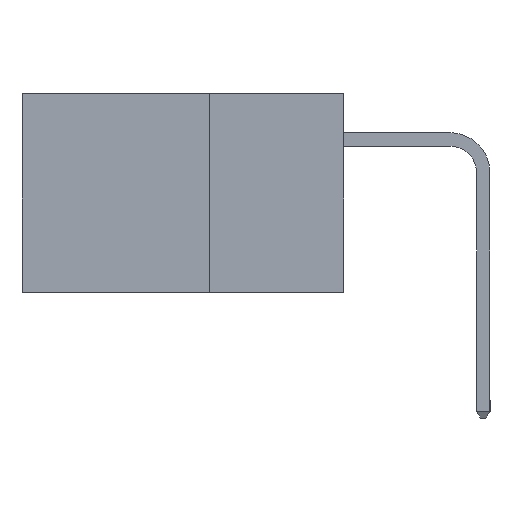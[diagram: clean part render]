
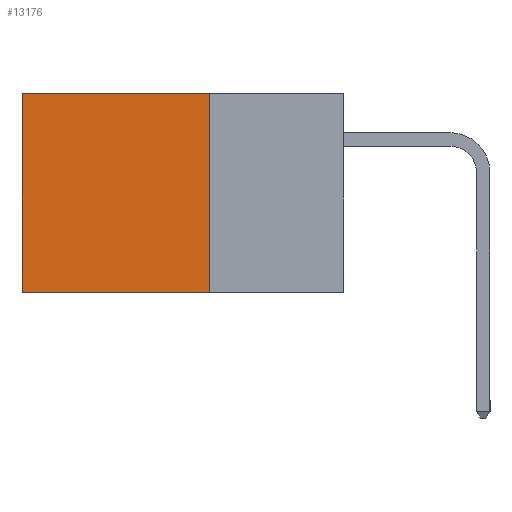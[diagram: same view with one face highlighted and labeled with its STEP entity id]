
A CAD part, left-side view. The second image highlights one B-rep face of the part: STEP entity #13176.
In plain terms, the highlighted planar face has unit normal (-1, 0, 0).
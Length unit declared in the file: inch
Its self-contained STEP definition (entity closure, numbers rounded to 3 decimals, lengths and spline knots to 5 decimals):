
#333 = CARTESIAN_POINT ( 'NONE',  ( 0.2615, 0.6, -0.37 ) ) ;
#347 = CARTESIAN_POINT ( 'NONE',  ( 0.2615, 0.25, 0. ) ) ;
#419 = DIRECTION ( 'NONE',  ( 0., 1., 0. ) ) ;
#1109 = DIRECTION ( 'NONE',  ( 1., 0., 0. ) ) ;
#2502 = VERTEX_POINT ( 'NONE', #6564 ) ;
#2642 = ORIENTED_EDGE ( 'NONE', *, *, #3732, .T. ) ;
#2700 = LINE ( 'NONE', #7761, #5968 ) ;
#2918 = VECTOR ( 'NONE', #11281, 39.37008 ) ;
#3124 = EDGE_CURVE ( 'NONE', #2502, #11687, #10125, .T. ) ;
#3251 = DIRECTION ( 'NONE',  ( 0., 0., -1. ) ) ;
#3732 = EDGE_CURVE ( 'NONE', #7903, #11687, #11468, .T. ) ;
#4304 = VECTOR ( 'NONE', #12937, 39.37008 ) ;
#5243 = PLANE ( 'NONE',  #12596 ) ;
#5786 = VECTOR ( 'NONE', #419, 39.37008 ) ;
#5968 = VECTOR ( 'NONE', #7655, 39.37008 ) ;
#6080 = CARTESIAN_POINT ( 'NONE',  ( 0.2615, 0.6, 0. ) ) ;
#6446 = CARTESIAN_POINT ( 'NONE',  ( 0.2615, 0.25, -0.37 ) ) ;
#6500 = ORIENTED_EDGE ( 'NONE', *, *, #3124, .F. ) ;
#6564 = CARTESIAN_POINT ( 'NONE',  ( 0.2615, 0.25, -0.37 ) ) ;
#7358 = EDGE_CURVE ( 'NONE', #10373, #2502, #2700, .T. ) ;
#7655 = DIRECTION ( 'NONE',  ( 0., 0., -1. ) ) ;
#7704 = FACE_OUTER_BOUND ( 'NONE', #12308, .T. ) ;
#7761 = CARTESIAN_POINT ( 'NONE',  ( 0.2615, 0.25, -0.37 ) ) ;
#7903 = VERTEX_POINT ( 'NONE', #6080 ) ;
#8422 = EDGE_CURVE ( 'NONE', #10373, #7903, #13322, .T. ) ;
#10125 = LINE ( 'NONE', #6446, #4304 ) ;
#10373 = VERTEX_POINT ( 'NONE', #11494 ) ;
#11281 = DIRECTION ( 'NONE',  ( 0., 0., -1. ) ) ;
#11468 = LINE ( 'NONE', #333, #2918 ) ;
#11494 = CARTESIAN_POINT ( 'NONE',  ( 0.2615, 0.25, 0. ) ) ;
#11687 = VERTEX_POINT ( 'NONE', #13494 ) ;
#12063 = ORIENTED_EDGE ( 'NONE', *, *, #8422, .T. ) ;
#12308 = EDGE_LOOP ( 'NONE', ( #2642, #6500, #12825, #12063 ) ) ;
#12596 = AXIS2_PLACEMENT_3D ( 'NONE', #12908, #1109, #3251 ) ;
#12825 = ORIENTED_EDGE ( 'NONE', *, *, #7358, .F. ) ;
#12908 = CARTESIAN_POINT ( 'NONE',  ( 0.2615, 0.25, -0.37 ) ) ;
#12937 = DIRECTION ( 'NONE',  ( 0., 1., 0. ) ) ;
#13176 = ADVANCED_FACE ( 'NONE', ( #7704 ), #5243, .F. ) ;
#13322 = LINE ( 'NONE', #347, #5786 ) ;
#13494 = CARTESIAN_POINT ( 'NONE',  ( 0.2615, 0.6, -0.37 ) ) ;
